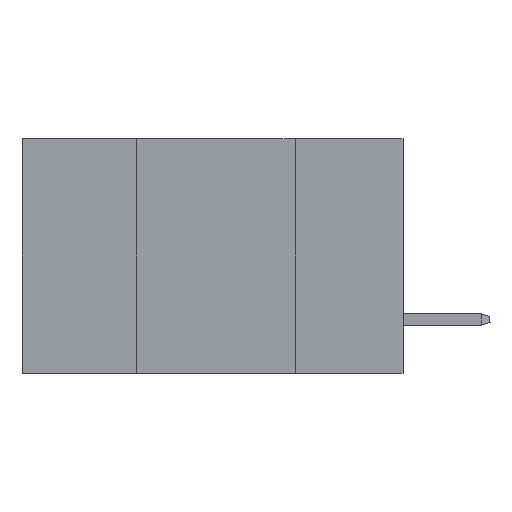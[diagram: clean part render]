
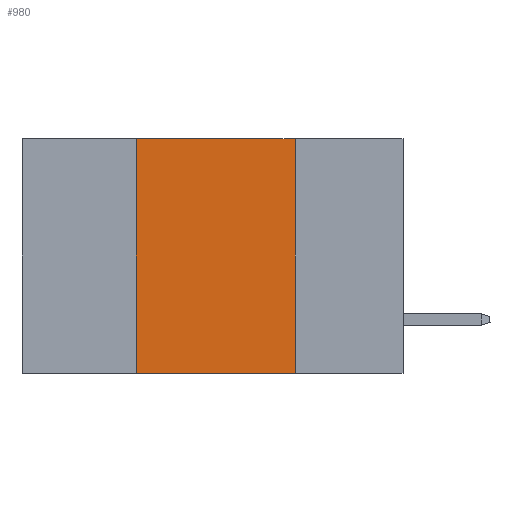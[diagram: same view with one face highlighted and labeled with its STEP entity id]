
A CAD part, left-side view. The second image highlights one B-rep face of the part: STEP entity #980.
In plain terms, the highlighted planar face has unit normal (-1, 0, 0).
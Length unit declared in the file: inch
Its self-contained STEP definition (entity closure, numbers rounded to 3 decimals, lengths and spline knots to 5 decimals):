
#364 = AXIS2_PLACEMENT_3D ( 'NONE', #10772, #15705, #18645 ) ;
#980 = ADVANCED_FACE ( 'NONE', ( #12395 ), #20529, .F. ) ;
#1119 = ORIENTED_EDGE ( 'NONE', *, *, #18462, .F. ) ;
#2076 = VERTEX_POINT ( 'NONE', #3838 ) ;
#2179 = LINE ( 'NONE', #11849, #19699 ) ;
#3721 = VECTOR ( 'NONE', #11643, 39.37008 ) ;
#3830 = LINE ( 'NONE', #10432, #8616 ) ;
#3838 = CARTESIAN_POINT ( 'NONE',  ( 0., 0.42, 0. ) ) ;
#3889 = DIRECTION ( 'NONE',  ( 0., -1., 0. ) ) ;
#4326 = LINE ( 'NONE', #5473, #10400 ) ;
#5473 = CARTESIAN_POINT ( 'NONE',  ( 0., 0.17, 0. ) ) ;
#6393 = VERTEX_POINT ( 'NONE', #20299 ) ;
#8331 = EDGE_CURVE ( 'NONE', #6393, #16597, #3830, .T. ) ;
#8616 = VECTOR ( 'NONE', #16765, 39.37008 ) ;
#10400 = VECTOR ( 'NONE', #14942, 39.37008 ) ;
#10432 = CARTESIAN_POINT ( 'NONE',  ( 0., 0.6, -0.37 ) ) ;
#10772 = CARTESIAN_POINT ( 'NONE',  ( 0., 0.6, 0. ) ) ;
#11342 = ORIENTED_EDGE ( 'NONE', *, *, #18090, .F. ) ;
#11566 = VERTEX_POINT ( 'NONE', #20163 ) ;
#11643 = DIRECTION ( 'NONE',  ( 0., 0., 1. ) ) ;
#11849 = CARTESIAN_POINT ( 'NONE',  ( 0., 0.6, 0. ) ) ;
#12395 = FACE_OUTER_BOUND ( 'NONE', #19535, .T. ) ;
#14622 = LINE ( 'NONE', #16414, #3721 ) ;
#14942 = DIRECTION ( 'NONE',  ( 0., 0., -1. ) ) ;
#15705 = DIRECTION ( 'NONE',  ( 1., 0., 0. ) ) ;
#15990 = ORIENTED_EDGE ( 'NONE', *, *, #8331, .T. ) ;
#16414 = CARTESIAN_POINT ( 'NONE',  ( 0., 0.42, 0. ) ) ;
#16597 = VERTEX_POINT ( 'NONE', #18221 ) ;
#16765 = DIRECTION ( 'NONE',  ( 0., -1., 0. ) ) ;
#18090 = EDGE_CURVE ( 'NONE', #11566, #16597, #4326, .T. ) ;
#18165 = ORIENTED_EDGE ( 'NONE', *, *, #18361, .F. ) ;
#18221 = CARTESIAN_POINT ( 'NONE',  ( 0., 0.17, -0.37 ) ) ;
#18361 = EDGE_CURVE ( 'NONE', #6393, #2076, #14622, .T. ) ;
#18462 = EDGE_CURVE ( 'NONE', #2076, #11566, #2179, .T. ) ;
#18645 = DIRECTION ( 'NONE',  ( 0., 0., -1. ) ) ;
#19535 = EDGE_LOOP ( 'NONE', ( #11342, #1119, #18165, #15990 ) ) ;
#19699 = VECTOR ( 'NONE', #3889, 39.37008 ) ;
#20163 = CARTESIAN_POINT ( 'NONE',  ( 0., 0.17, 0. ) ) ;
#20299 = CARTESIAN_POINT ( 'NONE',  ( 0., 0.42, -0.37 ) ) ;
#20529 = PLANE ( 'NONE',  #364 ) ;
